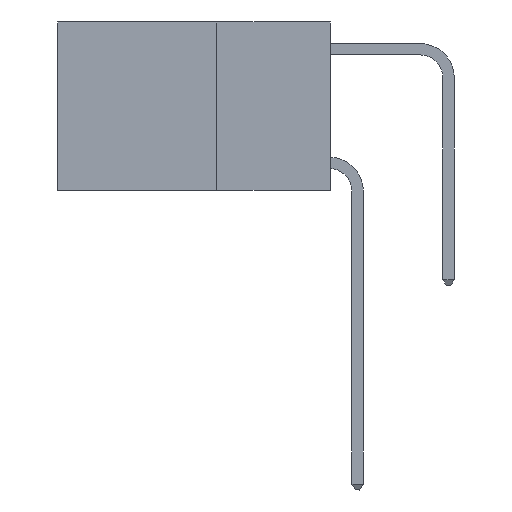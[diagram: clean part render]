
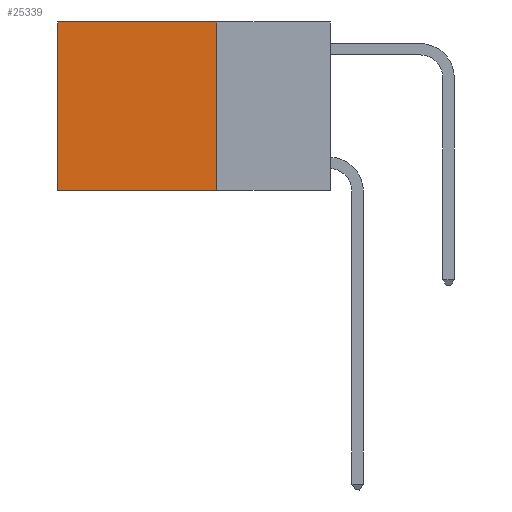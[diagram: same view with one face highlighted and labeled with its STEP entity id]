
A CAD part, left-side view. The second image highlights one B-rep face of the part: STEP entity #25339.
In plain terms, the highlighted planar face has unit normal (-1, 0, 0).
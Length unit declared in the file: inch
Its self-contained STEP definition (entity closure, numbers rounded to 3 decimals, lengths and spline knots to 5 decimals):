
#1948 = VECTOR ( 'NONE', #4247, 39.37008 ) ;
#2599 = LINE ( 'NONE', #19334, #8426 ) ;
#2961 = ORIENTED_EDGE ( 'NONE', *, *, #17947, .T. ) ;
#3593 = PLANE ( 'NONE',  #20435 ) ;
#4247 = DIRECTION ( 'NONE',  ( 0., 1., 0. ) ) ;
#4313 = EDGE_CURVE ( 'NONE', #8094, #5379, #5969, .T. ) ;
#5379 = VERTEX_POINT ( 'NONE', #5735 ) ;
#5441 = CARTESIAN_POINT ( 'NONE',  ( 0.2625, 0.6, -0.37 ) ) ;
#5735 = CARTESIAN_POINT ( 'NONE',  ( 0.2625, 0.25, -0.37 ) ) ;
#5969 = LINE ( 'NONE', #8064, #9399 ) ;
#7628 = CARTESIAN_POINT ( 'NONE',  ( 0.2625, 0.25, 0. ) ) ;
#8064 = CARTESIAN_POINT ( 'NONE',  ( 0.2625, 0.25, 0. ) ) ;
#8094 = VERTEX_POINT ( 'NONE', #22478 ) ;
#8426 = VECTOR ( 'NONE', #25685, 39.37008 ) ;
#9399 = VECTOR ( 'NONE', #20473, 39.37008 ) ;
#9545 = ORIENTED_EDGE ( 'NONE', *, *, #4313, .F. ) ;
#11512 = FACE_OUTER_BOUND ( 'NONE', #13343, .T. ) ;
#11931 = DIRECTION ( 'NONE',  ( 0., 0., -1. ) ) ;
#12561 = VECTOR ( 'NONE', #18389, 39.37008 ) ;
#13343 = EDGE_LOOP ( 'NONE', ( #17694, #18762, #9545, #2961 ) ) ;
#14662 = CARTESIAN_POINT ( 'NONE',  ( 0.2625, 0.6, 0. ) ) ;
#15193 = CARTESIAN_POINT ( 'NONE',  ( 0.2625, 0.6, 0. ) ) ;
#15464 = VERTEX_POINT ( 'NONE', #5441 ) ;
#17694 = ORIENTED_EDGE ( 'NONE', *, *, #25581, .T. ) ;
#17947 = EDGE_CURVE ( 'NONE', #8094, #20379, #18905, .T. ) ;
#17995 = DIRECTION ( 'NONE',  ( 1., 0., 0. ) ) ;
#18389 = DIRECTION ( 'NONE',  ( 0., 0., -1. ) ) ;
#18762 = ORIENTED_EDGE ( 'NONE', *, *, #19930, .F. ) ;
#18905 = LINE ( 'NONE', #21103, #1948 ) ;
#19334 = CARTESIAN_POINT ( 'NONE',  ( 0.2625, 0.25, -0.37 ) ) ;
#19930 = EDGE_CURVE ( 'NONE', #5379, #15464, #2599, .T. ) ;
#20379 = VERTEX_POINT ( 'NONE', #15193 ) ;
#20435 = AXIS2_PLACEMENT_3D ( 'NONE', #7628, #17995, #11931 ) ;
#20473 = DIRECTION ( 'NONE',  ( 0., 0., -1. ) ) ;
#21103 = CARTESIAN_POINT ( 'NONE',  ( 0.2625, 0.25, 0. ) ) ;
#22478 = CARTESIAN_POINT ( 'NONE',  ( 0.2625, 0.25, 0. ) ) ;
#22934 = LINE ( 'NONE', #14662, #12561 ) ;
#25339 = ADVANCED_FACE ( 'NONE', ( #11512 ), #3593, .F. ) ;
#25581 = EDGE_CURVE ( 'NONE', #20379, #15464, #22934, .T. ) ;
#25685 = DIRECTION ( 'NONE',  ( 0., 1., 0. ) ) ;
